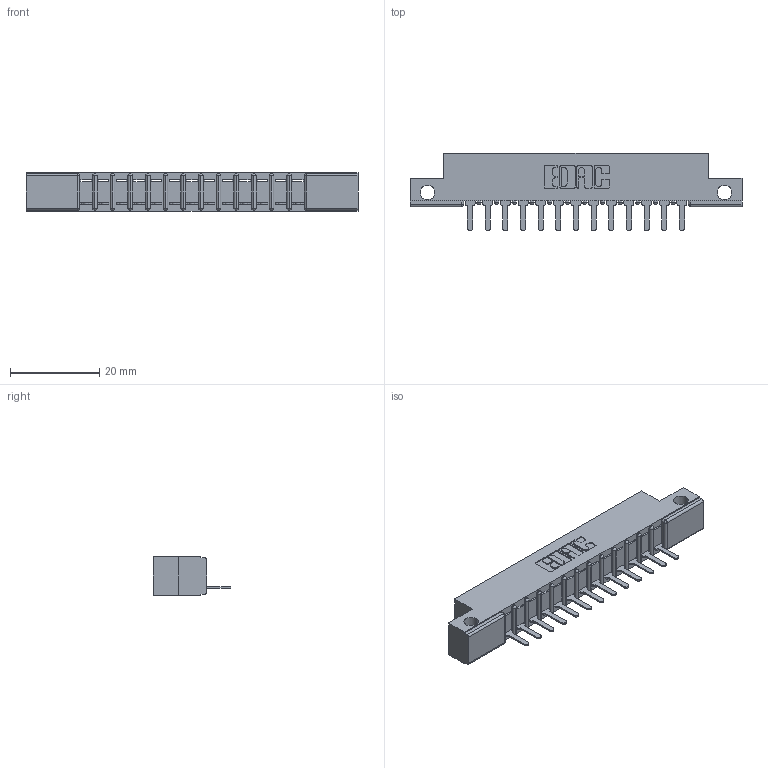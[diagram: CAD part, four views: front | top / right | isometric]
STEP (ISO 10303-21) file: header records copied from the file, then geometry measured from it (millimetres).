
FILE_DESCRIPTION (( 'STEP AP203' ), '1' );
FILE_NAME ('307-013-425-112.STEP', '2020-09-25T12:50:54', ( '' ), ( '' ), 'SwSTEP 2.0', 'SolidWorks 2020', '' );
FILE_SCHEMA (( 'CONFIG_CONTROL_DESIGN' ));
Length unit declared in the file: inch
Products named in the file (7): 307-013-425-112; 307 Part_.128 Dia Side Mounting Holes; 307-290-001_525; #15628; 307 Part_No Mounting Lugs; 307-013-427-101; 307-290-001_527
Assembly tree (14 placements, depth 2):
  307-013-425-112
    307 Part_.128 Dia Side Mounting Holes
    307-290-001_525  x13
  #15628
  307 Part_No Mounting Lugs
  307-013-427-101
  307-290-001_527
Bounding box: 74.52 x 17.42 x 8.71 mm (x, y, z)
Volume: 4641.6 mm3; surface area: 6636.1 mm2
Topology: 14 solids, 14 shells, 860 faces, 2429 edges, 1562 vertices
Faces by surface type: plane 551, cylinder 281, sphere 28
Entity records: 35823 total; most frequent: CARTESIAN_POINT 6042, ORIENTED_EDGE 5963, DIRECTION 5832, EDGE_CURVE 2966, VECTOR 2273, LINE 2241, VERTEX_POINT 1926, AXIS2_PLACEMENT_3D 1780
